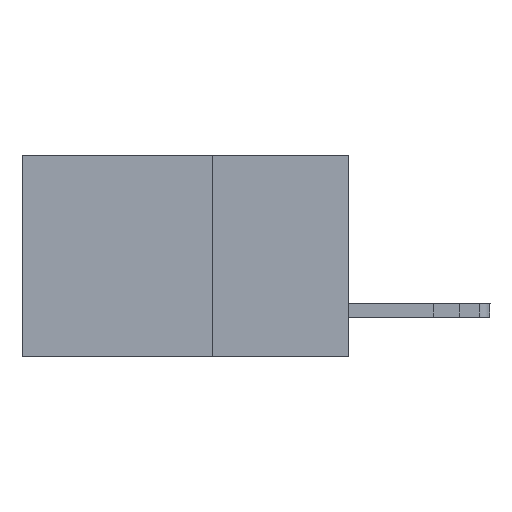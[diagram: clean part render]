
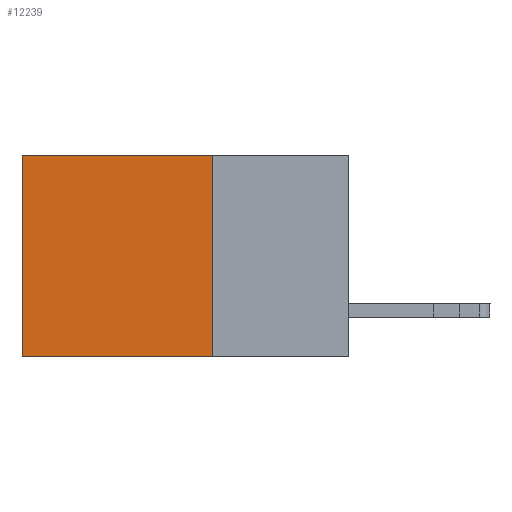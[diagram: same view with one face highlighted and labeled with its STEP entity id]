
A CAD part, left-side view. The second image highlights one B-rep face of the part: STEP entity #12239.
In plain terms, the highlighted planar face has unit normal (-1, 0, 0).
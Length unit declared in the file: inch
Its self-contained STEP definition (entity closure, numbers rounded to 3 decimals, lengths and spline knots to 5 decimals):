
#493 = CARTESIAN_POINT ( 'NONE',  ( 0.2615, 0.25, -0.37 ) ) ;
#525 = FACE_OUTER_BOUND ( 'NONE', #4993, .T. ) ;
#1230 = VERTEX_POINT ( 'NONE', #12190 ) ;
#1456 = EDGE_CURVE ( 'NONE', #10188, #11645, #3712, .T. ) ;
#1950 = CARTESIAN_POINT ( 'NONE',  ( 0.2615, 0.25, -0.37 ) ) ;
#2901 = ORIENTED_EDGE ( 'NONE', *, *, #4687, .T. ) ;
#3437 = LINE ( 'NONE', #11381, #5807 ) ;
#3712 = LINE ( 'NONE', #493, #8323 ) ;
#4138 = VECTOR ( 'NONE', #7542, 39.37008 ) ;
#4687 = EDGE_CURVE ( 'NONE', #1230, #8534, #12344, .T. ) ;
#4993 = EDGE_LOOP ( 'NONE', ( #5103, #10208, #5764, #2901 ) ) ;
#5103 = ORIENTED_EDGE ( 'NONE', *, *, #12330, .T. ) ;
#5764 = ORIENTED_EDGE ( 'NONE', *, *, #11510, .F. ) ;
#5807 = VECTOR ( 'NONE', #12414, 39.37008 ) ;
#6111 = DIRECTION ( 'NONE',  ( 1., 0., 0. ) ) ;
#6361 = CARTESIAN_POINT ( 'NONE',  ( 0.2615, 0.25, -0.37 ) ) ;
#7046 = CARTESIAN_POINT ( 'NONE',  ( 0.2615, 0.25, 0. ) ) ;
#7066 = DIRECTION ( 'NONE',  ( 0., 0., -1. ) ) ;
#7542 = DIRECTION ( 'NONE',  ( 0., 0., -1. ) ) ;
#8323 = VECTOR ( 'NONE', #9529, 39.37008 ) ;
#8534 = VERTEX_POINT ( 'NONE', #8739 ) ;
#8649 = AXIS2_PLACEMENT_3D ( 'NONE', #10445, #6111, #7066 ) ;
#8739 = CARTESIAN_POINT ( 'NONE',  ( 0.2615, 0.6, 0. ) ) ;
#9529 = DIRECTION ( 'NONE',  ( 0., 1., 0. ) ) ;
#9822 = LINE ( 'NONE', #1950, #4138 ) ;
#10188 = VERTEX_POINT ( 'NONE', #6361 ) ;
#10208 = ORIENTED_EDGE ( 'NONE', *, *, #1456, .F. ) ;
#10445 = CARTESIAN_POINT ( 'NONE',  ( 0.2615, 0.25, -0.37 ) ) ;
#11351 = CARTESIAN_POINT ( 'NONE',  ( 0.2615, 0.6, -0.37 ) ) ;
#11381 = CARTESIAN_POINT ( 'NONE',  ( 0.2615, 0.6, -0.37 ) ) ;
#11510 = EDGE_CURVE ( 'NONE', #1230, #10188, #9822, .T. ) ;
#11553 = PLANE ( 'NONE',  #8649 ) ;
#11621 = VECTOR ( 'NONE', #12636, 39.37008 ) ;
#11645 = VERTEX_POINT ( 'NONE', #11351 ) ;
#12190 = CARTESIAN_POINT ( 'NONE',  ( 0.2615, 0.25, 0. ) ) ;
#12239 = ADVANCED_FACE ( 'NONE', ( #525 ), #11553, .F. ) ;
#12330 = EDGE_CURVE ( 'NONE', #8534, #11645, #3437, .T. ) ;
#12344 = LINE ( 'NONE', #7046, #11621 ) ;
#12414 = DIRECTION ( 'NONE',  ( 0., 0., -1. ) ) ;
#12636 = DIRECTION ( 'NONE',  ( 0., 1., 0. ) ) ;
